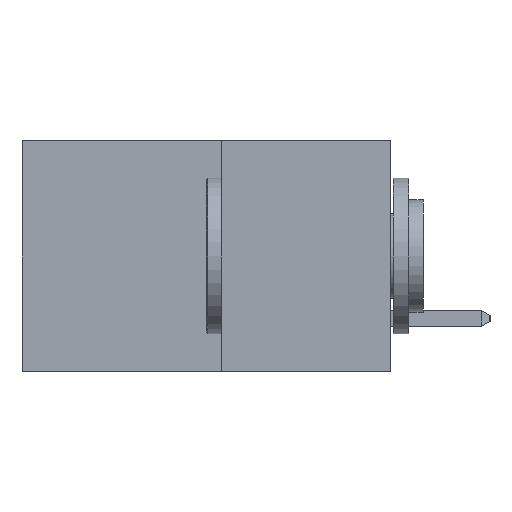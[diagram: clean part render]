
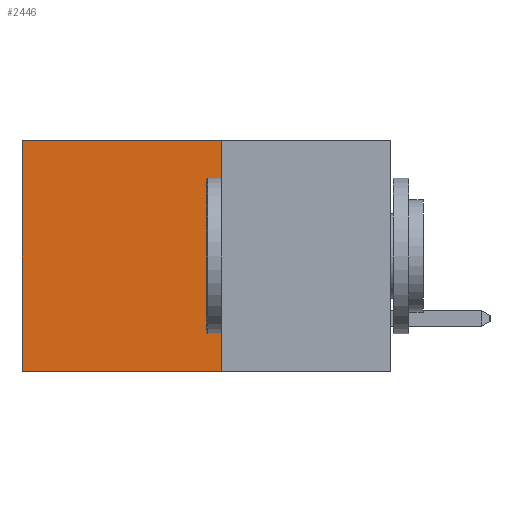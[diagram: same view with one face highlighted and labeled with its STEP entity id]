
A CAD part, left-side view. The second image highlights one B-rep face of the part: STEP entity #2446.
In plain terms, the highlighted planar face has unit normal (-1, 0, 0).
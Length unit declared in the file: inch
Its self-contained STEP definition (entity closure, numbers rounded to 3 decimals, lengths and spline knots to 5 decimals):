
#422 = LINE ( 'NONE', #1970, #6205 ) ;
#1018 = EDGE_CURVE ( 'NONE', #2094, #7573, #8721, .T. ) ;
#1463 = DIRECTION ( 'NONE',  ( 0., 0., -1. ) ) ;
#1934 = DIRECTION ( 'NONE',  ( 0., 0., -1. ) ) ;
#1970 = CARTESIAN_POINT ( 'NONE',  ( 0.277, 0.59, -0.37 ) ) ;
#2094 = VERTEX_POINT ( 'NONE', #8125 ) ;
#2446 = ADVANCED_FACE ( 'NONE', ( #8278 ), #7421, .F. ) ;
#2681 = VECTOR ( 'NONE', #3610, 39.37008 ) ;
#3338 = LINE ( 'NONE', #6195, #9308 ) ;
#3495 = DIRECTION ( 'NONE',  ( 0., 0., -1. ) ) ;
#3610 = DIRECTION ( 'NONE',  ( 0., 1., 0. ) ) ;
#3843 = EDGE_LOOP ( 'NONE', ( #4529, #5320, #4733, #5808 ) ) ;
#4529 = ORIENTED_EDGE ( 'NONE', *, *, #6450, .T. ) ;
#4733 = ORIENTED_EDGE ( 'NONE', *, *, #9008, .F. ) ;
#5320 = ORIENTED_EDGE ( 'NONE', *, *, #9731, .F. ) ;
#5773 = CARTESIAN_POINT ( 'NONE',  ( 0.277, 0.27, 0. ) ) ;
#5808 = ORIENTED_EDGE ( 'NONE', *, *, #1018, .T. ) ;
#6195 = CARTESIAN_POINT ( 'NONE',  ( 0.277, 0.27, -0.37 ) ) ;
#6205 = VECTOR ( 'NONE', #1934, 39.37008 ) ;
#6450 = EDGE_CURVE ( 'NONE', #7573, #6777, #422, .T. ) ;
#6720 = CARTESIAN_POINT ( 'NONE',  ( 0.277, 0.27, -0.37 ) ) ;
#6777 = VERTEX_POINT ( 'NONE', #9790 ) ;
#7053 = CARTESIAN_POINT ( 'NONE',  ( 0.277, 0.27, -0.37 ) ) ;
#7179 = DIRECTION ( 'NONE',  ( 1., 0., 0. ) ) ;
#7421 = PLANE ( 'NONE',  #8234 ) ;
#7573 = VERTEX_POINT ( 'NONE', #7900 ) ;
#7777 = DIRECTION ( 'NONE',  ( 0., 1., 0. ) ) ;
#7900 = CARTESIAN_POINT ( 'NONE',  ( 0.277, 0.59, 0. ) ) ;
#8116 = VERTEX_POINT ( 'NONE', #8525 ) ;
#8125 = CARTESIAN_POINT ( 'NONE',  ( 0.277, 0.27, 0. ) ) ;
#8204 = VECTOR ( 'NONE', #7777, 39.37008 ) ;
#8234 = AXIS2_PLACEMENT_3D ( 'NONE', #6720, #7179, #3495 ) ;
#8278 = FACE_OUTER_BOUND ( 'NONE', #3843, .T. ) ;
#8433 = LINE ( 'NONE', #7053, #8204 ) ;
#8525 = CARTESIAN_POINT ( 'NONE',  ( 0.277, 0.27, -0.37 ) ) ;
#8721 = LINE ( 'NONE', #5773, #2681 ) ;
#9008 = EDGE_CURVE ( 'NONE', #2094, #8116, #3338, .T. ) ;
#9308 = VECTOR ( 'NONE', #1463, 39.37008 ) ;
#9731 = EDGE_CURVE ( 'NONE', #8116, #6777, #8433, .T. ) ;
#9790 = CARTESIAN_POINT ( 'NONE',  ( 0.277, 0.59, -0.37 ) ) ;
